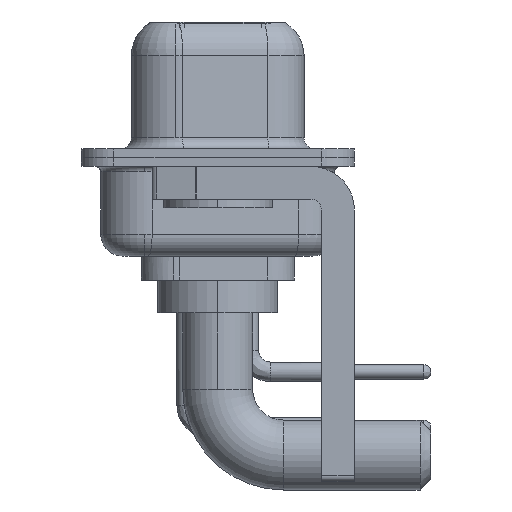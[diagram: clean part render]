
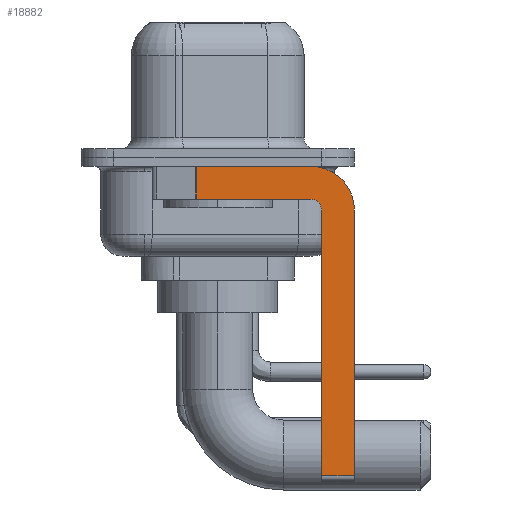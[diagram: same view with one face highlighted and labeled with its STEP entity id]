
A CAD part, left-side view. The second image highlights one B-rep face of the part: STEP entity #18882.
In plain terms, the highlighted planar face has unit normal (-1, 0, 0).
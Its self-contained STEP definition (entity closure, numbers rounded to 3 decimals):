
#147 = ORIENTED_EDGE ( 'NONE', *, *, #11656, .T. ) ;
#247 = CARTESIAN_POINT ( 'NONE',  ( -2.9, -6.25, -14.55 ) ) ;
#510 = CARTESIAN_POINT ( 'NONE',  ( -2.9, -4.75, -14.55 ) ) ;
#1619 = LINE ( 'NONE', #14462, #4002 ) ;
#1948 = LINE ( 'NONE', #9994, #20757 ) ;
#2052 = CARTESIAN_POINT ( 'NONE',  ( -2.9, -4.25, -0.4 ) ) ;
#2419 = EDGE_CURVE ( 'NONE', #8070, #17490, #20738, .T. ) ;
#2549 = ORIENTED_EDGE ( 'NONE', *, *, #20379, .T. ) ;
#3320 = LINE ( 'NONE', #17965, #9238 ) ;
#3552 = CIRCLE ( 'NONE', #5933, 0.5 ) ;
#4002 = VECTOR ( 'NONE', #11168, 1000. ) ;
#4006 = EDGE_CURVE ( 'NONE', #13469, #12493, #4950, .T. ) ;
#4211 = VERTEX_POINT ( 'NONE', #14507 ) ;
#4334 = LINE ( 'NONE', #7724, #14629 ) ;
#4829 = PLANE ( 'NONE',  #16866 ) ;
#4950 = CIRCLE ( 'NONE', #5289, 2. ) ;
#5289 = AXIS2_PLACEMENT_3D ( 'NONE', #19694, #16539, #6870 ) ;
#5548 = CARTESIAN_POINT ( 'NONE',  ( -2.9, -4.25, -2.4 ) ) ;
#5615 = EDGE_CURVE ( 'NONE', #11942, #13469, #1619, .T. ) ;
#5670 = ORIENTED_EDGE ( 'NONE', *, *, #5615, .F. ) ;
#5933 = AXIS2_PLACEMENT_3D ( 'NONE', #5548, #10111, #9997 ) ;
#6616 = DIRECTION ( 'NONE',  ( 0., -1., 0. ) ) ;
#6870 = DIRECTION ( 'NONE',  ( 0., 0., -1. ) ) ;
#7724 = CARTESIAN_POINT ( 'NONE',  ( -2.9, -4.25, -1.9 ) ) ;
#7958 = CARTESIAN_POINT ( 'NONE',  ( -2.9, 0.978, -0.4 ) ) ;
#8012 = CARTESIAN_POINT ( 'NONE',  ( -2.9, -4.25, -2.4 ) ) ;
#8070 = VERTEX_POINT ( 'NONE', #510 ) ;
#8248 = VERTEX_POINT ( 'NONE', #9720 ) ;
#9098 = ORIENTED_EDGE ( 'NONE', *, *, #14884, .F. ) ;
#9112 = DIRECTION ( 'NONE',  ( 0., 0., -1. ) ) ;
#9238 = VECTOR ( 'NONE', #11181, 1000. ) ;
#9720 = CARTESIAN_POINT ( 'NONE',  ( -2.9, 0.978, -1.9 ) ) ;
#9799 = VECTOR ( 'NONE', #9112, 1000. ) ;
#9994 = CARTESIAN_POINT ( 'NONE',  ( -2.9, -4.25, -14.55 ) ) ;
#9997 = DIRECTION ( 'NONE',  ( 0., 0., 1. ) ) ;
#10111 = DIRECTION ( 'NONE',  ( -1., 0., 0. ) ) ;
#10882 = DIRECTION ( 'NONE',  ( 0., 0., -1. ) ) ;
#11034 = EDGE_CURVE ( 'NONE', #4211, #8248, #4334, .T. ) ;
#11168 = DIRECTION ( 'NONE',  ( 0., -1., 0. ) ) ;
#11181 = DIRECTION ( 'NONE',  ( 0., 0., -1. ) ) ;
#11656 = EDGE_CURVE ( 'NONE', #8070, #19615, #1948, .T. ) ;
#11942 = VERTEX_POINT ( 'NONE', #7958 ) ;
#12493 = VERTEX_POINT ( 'NONE', #15812 ) ;
#12589 = CARTESIAN_POINT ( 'NONE',  ( -2.9, -4.75, -14.8 ) ) ;
#13242 = EDGE_CURVE ( 'NONE', #12493, #19615, #3320, .T. ) ;
#13469 = VERTEX_POINT ( 'NONE', #2052 ) ;
#14214 = DIRECTION ( 'NONE',  ( 0., 1., 0. ) ) ;
#14257 = ORIENTED_EDGE ( 'NONE', *, *, #13242, .F. ) ;
#14462 = CARTESIAN_POINT ( 'NONE',  ( -2.9, 3., -0.4 ) ) ;
#14506 = FACE_OUTER_BOUND ( 'NONE', #17434, .T. ) ;
#14507 = CARTESIAN_POINT ( 'NONE',  ( -2.9, -4.25, -1.9 ) ) ;
#14514 = ORIENTED_EDGE ( 'NONE', *, *, #2419, .F. ) ;
#14629 = VECTOR ( 'NONE', #14214, 1000. ) ;
#14884 = EDGE_CURVE ( 'NONE', #17490, #4211, #3552, .T. ) ;
#15775 = DIRECTION ( 'NONE',  ( 0., 0., 1. ) ) ;
#15812 = CARTESIAN_POINT ( 'NONE',  ( -2.9, -6.25, -2.4 ) ) ;
#15923 = LINE ( 'NONE', #17185, #9799 ) ;
#16539 = DIRECTION ( 'NONE',  ( 1., 0., 0. ) ) ;
#16866 = AXIS2_PLACEMENT_3D ( 'NONE', #8012, #20855, #10882 ) ;
#17185 = CARTESIAN_POINT ( 'NONE',  ( -2.9, 0.978, -1.9 ) ) ;
#17434 = EDGE_LOOP ( 'NONE', ( #5670, #2549, #19250, #9098, #14514, #147, #14257, #20183 ) ) ;
#17490 = VERTEX_POINT ( 'NONE', #18195 ) ;
#17965 = CARTESIAN_POINT ( 'NONE',  ( -2.9, -6.25, -2.4 ) ) ;
#18195 = CARTESIAN_POINT ( 'NONE',  ( -2.9, -4.75, -2.4 ) ) ;
#18882 = ADVANCED_FACE ( 'NONE', ( #14506 ), #4829, .F. ) ;
#19250 = ORIENTED_EDGE ( 'NONE', *, *, #11034, .F. ) ;
#19615 = VERTEX_POINT ( 'NONE', #247 ) ;
#19694 = CARTESIAN_POINT ( 'NONE',  ( -2.9, -4.25, -2.4 ) ) ;
#19794 = VECTOR ( 'NONE', #15775, 1000. ) ;
#20183 = ORIENTED_EDGE ( 'NONE', *, *, #4006, .F. ) ;
#20379 = EDGE_CURVE ( 'NONE', #11942, #8248, #15923, .T. ) ;
#20738 = LINE ( 'NONE', #12589, #19794 ) ;
#20757 = VECTOR ( 'NONE', #6616, 1000. ) ;
#20855 = DIRECTION ( 'NONE',  ( 1., 0., 0. ) ) ;
